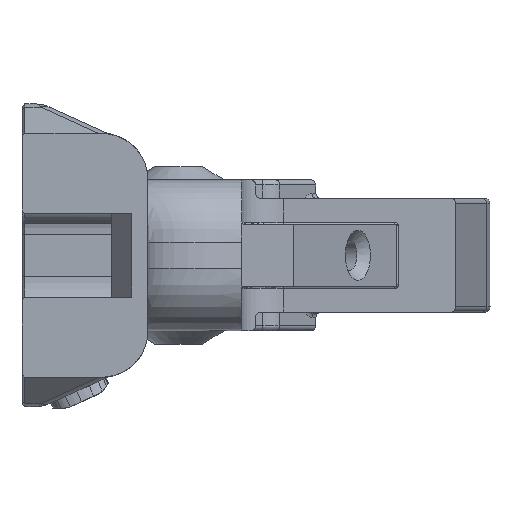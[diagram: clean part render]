
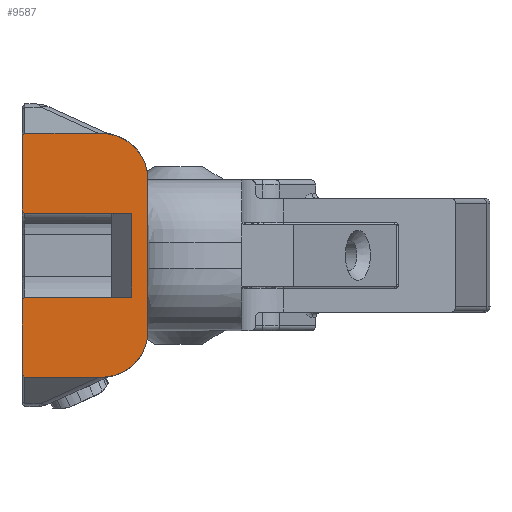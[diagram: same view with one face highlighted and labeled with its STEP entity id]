
A CAD part, left-side view. The second image highlights one B-rep face of the part: STEP entity #9587.
In plain terms, the highlighted planar face has unit normal (-1, 0, 0).
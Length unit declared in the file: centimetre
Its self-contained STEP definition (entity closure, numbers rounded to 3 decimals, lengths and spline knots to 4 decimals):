
#830=PLANE($,#10344);
#1411=FACE_OUTER_BOUND($,#2042,.T.);
#2042=EDGE_LOOP($,(#8846,#8847,#8848,#8849,#8850,#8851,#8852,#8853,#8854,
#8855,#8856,#8857,#8858,#8859));
#2136=CIRCLE($,#9754,0.7057);
#2346=CIRCLE($,#10345,0.7057);
#2413=LINE($,#13094,#3091);
#2424=LINE($,#13224,#3102);
#2989=LINE($,#22759,#3667);
#2991=LINE($,#22763,#3669);
#2993=LINE($,#22767,#3671);
#2995=LINE($,#22771,#3673);
#2997=LINE($,#22774,#3675);
#2998=LINE($,#22776,#3676);
#3000=LINE($,#22780,#3678);
#3002=LINE($,#22784,#3680);
#3004=LINE($,#22787,#3682);
#3021=LINE($,#23783,#3699);
#3091=VECTOR($,#10584,1.172);
#3102=VECTOR($,#10649,1.172);
#3667=VECTOR($,#12418,1.63);
#3669=VECTOR($,#12422,0.0566);
#3671=VECTOR($,#12426,0.0566);
#3673=VECTOR($,#12430,0.0566);
#3675=VECTOR($,#12434,1.1417);
#3676=VECTOR($,#12435,1.1417);
#3678=VECTOR($,#12439,0.0566);
#3680=VECTOR($,#12443,1.63);
#3682=VECTOR($,#12447,1.27);
#3699=VECTOR($,#12524,2.3019);
#3880=VERTEX_POINT($,#13091);
#3881=VERTEX_POINT($,#13093);
#3908=VERTEX_POINT($,#13221);
#3909=VERTEX_POINT($,#13223);
#3942=VERTEX_POINT($,#13710);
#4656=VERTEX_POINT($,#22756);
#4657=VERTEX_POINT($,#22758);
#4658=VERTEX_POINT($,#22762);
#4659=VERTEX_POINT($,#22766);
#4660=VERTEX_POINT($,#22770);
#4661=VERTEX_POINT($,#22775);
#4662=VERTEX_POINT($,#22779);
#4663=VERTEX_POINT($,#22783);
#4675=VERTEX_POINT($,#23782);
#4815=EDGE_CURVE($,#3880,#3881,#2413,.F.);
#4846=EDGE_CURVE($,#3908,#3909,#2424,.T.);
#4882=EDGE_CURVE($,#3942,#3908,#2136,.T.);
#6027=EDGE_CURVE($,#4656,#4657,#2989,.F.);
#6029=EDGE_CURVE($,#4657,#4658,#2991,.T.);
#6031=EDGE_CURVE($,#4659,#3880,#2993,.T.);
#6033=EDGE_CURVE($,#3909,#4660,#2995,.T.);
#6035=EDGE_CURVE($,#4658,#4659,#2997,.T.);
#6036=EDGE_CURVE($,#4660,#4661,#2998,.T.);
#6038=EDGE_CURVE($,#4661,#4662,#3000,.T.);
#6040=EDGE_CURVE($,#4662,#4663,#3002,.T.);
#6042=EDGE_CURVE($,#4663,#4656,#3004,.F.);
#6077=EDGE_CURVE($,#4675,#3942,#3021,.T.);
#6078=EDGE_CURVE($,#3881,#4675,#2346,.T.);
#8846=ORIENTED_EDGE($,*,*,#6042,.F.);
#8847=ORIENTED_EDGE($,*,*,#6040,.F.);
#8848=ORIENTED_EDGE($,*,*,#6038,.F.);
#8849=ORIENTED_EDGE($,*,*,#6036,.F.);
#8850=ORIENTED_EDGE($,*,*,#6033,.F.);
#8851=ORIENTED_EDGE($,*,*,#4846,.F.);
#8852=ORIENTED_EDGE($,*,*,#4882,.F.);
#8853=ORIENTED_EDGE($,*,*,#6077,.F.);
#8854=ORIENTED_EDGE($,*,*,#6078,.F.);
#8855=ORIENTED_EDGE($,*,*,#4815,.F.);
#8856=ORIENTED_EDGE($,*,*,#6031,.F.);
#8857=ORIENTED_EDGE($,*,*,#6035,.F.);
#8858=ORIENTED_EDGE($,*,*,#6029,.F.);
#8859=ORIENTED_EDGE($,*,*,#6027,.F.);
#9587=ADVANCED_FACE($,(#1411),#830,.F.);
#9754=AXIS2_PLACEMENT_3D($,#13712,#10752,#10753);
#10344=AXIS2_PLACEMENT_3D($,#23781,#12522,#12523);
#10345=AXIS2_PLACEMENT_3D($,#23784,#12525,#12526);
#10584=DIRECTION($,(0.,1.,0.));
#10649=DIRECTION($,(0.,1.,0.));
#10752=DIRECTION('center_axis',(1.,0.,0.));
#10753=DIRECTION('ref_axis',(0.,0.,
1.));
#12418=DIRECTION($,(0.,-1.,0.));
#12422=DIRECTION($,(0.,0.707,0.707));
#12426=DIRECTION($,(0.,-0.707,0.707));
#12430=DIRECTION($,(0.,0.707,0.707));
#12434=DIRECTION($,(0.,0.,1.));
#12435=DIRECTION($,(0.,0.,1.));
#12439=DIRECTION($,(0.,-0.707,0.707));
#12443=DIRECTION($,(0.,-1.,0.));
#12447=DIRECTION($,(0.,0.,-1.));
#12522=DIRECTION('center_axis',(1.,0.,0.));
#12523=DIRECTION('ref_axis',(0.,0.,
-1.));
#12524=DIRECTION($,(0.,0.,-1.));
#12525=DIRECTION('center_axis',(1.,0.,0.));
#12526=DIRECTION('ref_axis',(0.,0.,
1.));
#13091=CARTESIAN_POINT('',(-19.7417,0.5241,1.9567));
#13093=CARTESIAN_POINT('',(-19.7417,-0.6479,1.9567));
#13094=CARTESIAN_POINT($,(-19.7417,-0.2459,1.9567));
#13221=CARTESIAN_POINT('',(-19.7417,-0.6479,-1.7567));
#13223=CARTESIAN_POINT('',(-19.7417,0.5241,-1.7567));
#13224=CARTESIAN_POINT($,(-19.7417,0.1273,-1.7567));
#13710=CARTESIAN_POINT('',(-19.7417,-1.3536,-1.0509));
#13712=CARTESIAN_POINT('Origin',(-19.7417,-0.6479,-1.0509));
#22756=CARTESIAN_POINT('',(-19.7417,-1.1059,0.735));
#22758=CARTESIAN_POINT('',(-19.7417,0.5241,0.735));
#22759=CARTESIAN_POINT($,(-19.7417,1.81,0.735));
#22762=CARTESIAN_POINT('',(-19.7417,0.5641,0.775));
#22763=CARTESIAN_POINT($,(-19.7417,-0.1209,0.0901));
#22766=CARTESIAN_POINT('',(-19.7417,0.5641,1.9167));
#22767=CARTESIAN_POINT($,(-19.7417,1.0776,1.4031));
#22770=CARTESIAN_POINT('',(-19.7417,0.5641,-1.7167));
#22771=CARTESIAN_POINT($,(-19.7417,0.5021,-1.7787));
#22774=CARTESIAN_POINT($,(-19.7417,0.5641,-1.6584));
#22775=CARTESIAN_POINT('',(-19.7417,0.5641,-0.575));
#22776=CARTESIAN_POINT($,(-19.7417,0.5641,-1.6584));
#22779=CARTESIAN_POINT('',(-19.7417,0.5241,-0.535));
#22780=CARTESIAN_POINT($,(-19.7417,0.4547,-0.4656));
#22783=CARTESIAN_POINT('',(-19.7417,-1.1059,-0.535));
#22784=CARTESIAN_POINT($,(-19.7417,1.81,-0.535));
#22787=CARTESIAN_POINT($,(-19.7417,-1.1059,-0.4417));
#23781=CARTESIAN_POINT('Origin',(-19.7417,-0.3095,-1.0511));
#23782=CARTESIAN_POINT('',(-19.7417,-1.3536,1.2509));
#23783=CARTESIAN_POINT($,(-19.7417,-1.3536,-1.051));
#23784=CARTESIAN_POINT('Origin',(-19.7417,-0.6479,1.2509));
